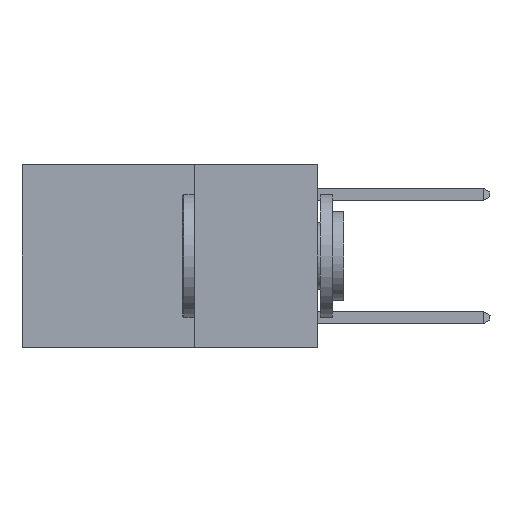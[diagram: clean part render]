
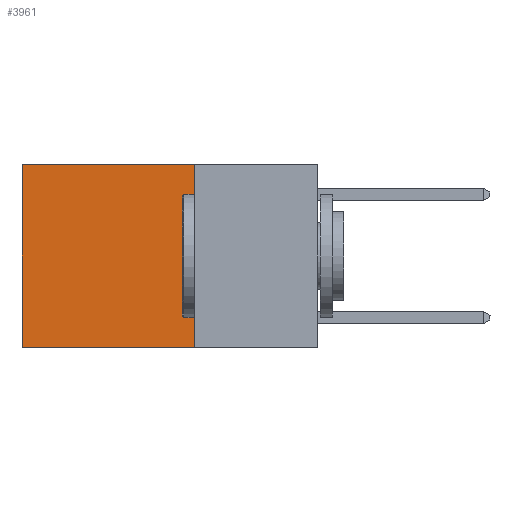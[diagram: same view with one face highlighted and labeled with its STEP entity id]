
A CAD part, left-side view. The second image highlights one B-rep face of the part: STEP entity #3961.
In plain terms, the highlighted planar face has unit normal (-1, 0, 0).
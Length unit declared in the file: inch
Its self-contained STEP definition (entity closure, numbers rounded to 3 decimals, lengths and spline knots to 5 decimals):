
#67 = LINE ( 'NONE', #2204, #11155 ) ;
#447 = VERTEX_POINT ( 'NONE', #6216 ) ;
#1604 = PLANE ( 'NONE',  #14904 ) ;
#2077 = DIRECTION ( 'NONE',  ( 0., 0., -1. ) ) ;
#2204 = CARTESIAN_POINT ( 'NONE',  ( 0.2625, 0.25, 0. ) ) ;
#2228 = EDGE_CURVE ( 'NONE', #16473, #447, #67, .T. ) ;
#3961 = ADVANCED_FACE ( 'NONE', ( #13965 ), #1604, .F. ) ;
#4552 = VECTOR ( 'NONE', #29767, 39.37008 ) ;
#5510 = CARTESIAN_POINT ( 'NONE',  ( 0.2625, 0.25, -0.37 ) ) ;
#6216 = CARTESIAN_POINT ( 'NONE',  ( 0.2625, 0.6, 0. ) ) ;
#6339 = DIRECTION ( 'NONE',  ( 1., 0., 0. ) ) ;
#6607 = ORIENTED_EDGE ( 'NONE', *, *, #2228, .T. ) ;
#6711 = LINE ( 'NONE', #12683, #25374 ) ;
#9346 = LINE ( 'NONE', #16167, #28675 ) ;
#10868 = LINE ( 'NONE', #18227, #4552 ) ;
#11155 = VECTOR ( 'NONE', #27961, 39.37008 ) ;
#12683 = CARTESIAN_POINT ( 'NONE',  ( 0.2625, 0.25, -0.37 ) ) ;
#13049 = CARTESIAN_POINT ( 'NONE',  ( 0.2625, 0.6, -0.37 ) ) ;
#13965 = FACE_OUTER_BOUND ( 'NONE', #25448, .T. ) ;
#14904 = AXIS2_PLACEMENT_3D ( 'NONE', #20352, #6339, #22692 ) ;
#16167 = CARTESIAN_POINT ( 'NONE',  ( 0.2625, 0.6, 0. ) ) ;
#16473 = VERTEX_POINT ( 'NONE', #28523 ) ;
#18227 = CARTESIAN_POINT ( 'NONE',  ( 0.2625, 0.25, 0. ) ) ;
#20352 = CARTESIAN_POINT ( 'NONE',  ( 0.2625, 0.25, 0. ) ) ;
#20591 = EDGE_CURVE ( 'NONE', #29474, #21401, #6711, .T. ) ;
#21401 = VERTEX_POINT ( 'NONE', #13049 ) ;
#22025 = DIRECTION ( 'NONE',  ( 0., 1., 0. ) ) ;
#22220 = ORIENTED_EDGE ( 'NONE', *, *, #25026, .F. ) ;
#22692 = DIRECTION ( 'NONE',  ( 0., 0., -1. ) ) ;
#23326 = ORIENTED_EDGE ( 'NONE', *, *, #25817, .T. ) ;
#25026 = EDGE_CURVE ( 'NONE', #16473, #29474, #10868, .T. ) ;
#25374 = VECTOR ( 'NONE', #22025, 39.37008 ) ;
#25448 = EDGE_LOOP ( 'NONE', ( #23326, #27943, #22220, #6607 ) ) ;
#25817 = EDGE_CURVE ( 'NONE', #447, #21401, #9346, .T. ) ;
#27943 = ORIENTED_EDGE ( 'NONE', *, *, #20591, .F. ) ;
#27961 = DIRECTION ( 'NONE',  ( 0., 1., 0. ) ) ;
#28523 = CARTESIAN_POINT ( 'NONE',  ( 0.2625, 0.25, 0. ) ) ;
#28675 = VECTOR ( 'NONE', #2077, 39.37008 ) ;
#29474 = VERTEX_POINT ( 'NONE', #5510 ) ;
#29767 = DIRECTION ( 'NONE',  ( 0., 0., -1. ) ) ;
